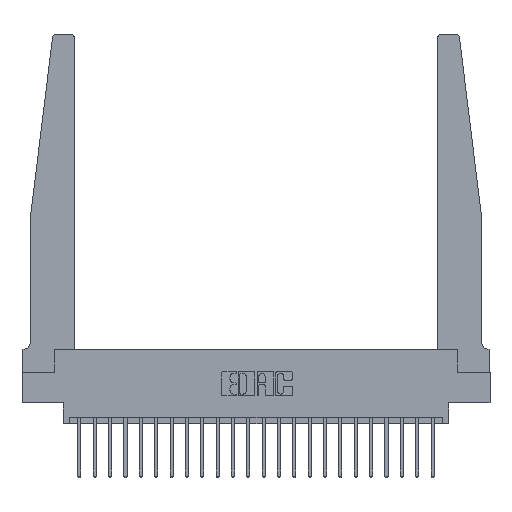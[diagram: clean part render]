
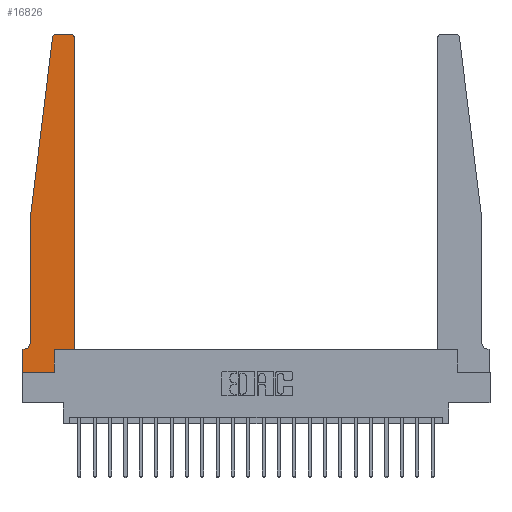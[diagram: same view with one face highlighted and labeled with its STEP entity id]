
A CAD part, top view. The second image highlights one B-rep face of the part: STEP entity #16826.
In plain terms, the highlighted planar face has unit normal (0, 0, 1).
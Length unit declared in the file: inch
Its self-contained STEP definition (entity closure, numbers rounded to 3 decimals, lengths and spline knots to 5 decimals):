
#52 = DIRECTION ( 'NONE',  ( -1., 0., 0. ) ) ;
#941 = EDGE_CURVE ( 'NONE', #4308, #5009, #6712, .T. ) ;
#975 = AXIS2_PLACEMENT_3D ( 'NONE', #16625, #5982, #18410 ) ;
#1387 = EDGE_CURVE ( 'NONE', #3531, #12288, #22010, .T. ) ;
#1699 = VECTOR ( 'NONE', #6866, 39.37008 ) ;
#2725 = VERTEX_POINT ( 'NONE', #20715 ) ;
#3095 = VECTOR ( 'NONE', #12484, 39.37008 ) ;
#3283 = LINE ( 'NONE', #10765, #21636 ) ;
#3531 = VERTEX_POINT ( 'NONE', #21065 ) ;
#3608 = EDGE_CURVE ( 'NONE', #15071, #17167, #10493, .T. ) ;
#3661 = CIRCLE ( 'NONE', #16187, 0.05 ) ;
#4035 = CARTESIAN_POINT ( 'NONE',  ( 0.2605, 0., 0.37 ) ) ;
#4235 = DIRECTION ( 'NONE',  ( 0., 0., 1. ) ) ;
#4308 = VERTEX_POINT ( 'NONE', #21750 ) ;
#4326 = CARTESIAN_POINT ( 'NONE',  ( 0.065, 0.1875, 0.37 ) ) ;
#4566 = DIRECTION ( 'NONE',  ( 0., 0., 1. ) ) ;
#4670 = CARTESIAN_POINT ( 'NONE',  ( 0.24675, 2.72367, 0.37 ) ) ;
#4792 = ORIENTED_EDGE ( 'NONE', *, *, #5842, .T. ) ;
#4995 = VECTOR ( 'NONE', #15937, 39.37008 ) ;
#5008 = CARTESIAN_POINT ( 'NONE',  ( 0.065, 0.2375, 0.37 ) ) ;
#5009 = VERTEX_POINT ( 'NONE', #4670 ) ;
#5294 = CARTESIAN_POINT ( 'NONE',  ( 0.2605, 0.18, 0.37 ) ) ;
#5448 = EDGE_CURVE ( 'NONE', #10392, #7543, #20905, .T. ) ;
#5519 = VECTOR ( 'NONE', #13654, 39.37008 ) ;
#5685 = EDGE_CURVE ( 'NONE', #8051, #8667, #15315, .T. ) ;
#5794 = ORIENTED_EDGE ( 'NONE', *, *, #17753, .T. ) ;
#5842 = EDGE_CURVE ( 'NONE', #12288, #10392, #3661, .T. ) ;
#5930 = CARTESIAN_POINT ( 'NONE',  ( 0., 0.1875, 0.37 ) ) ;
#5982 = DIRECTION ( 'NONE',  ( 0., 0., 1. ) ) ;
#6063 = ORIENTED_EDGE ( 'NONE', *, *, #5448, .T. ) ;
#6693 = CIRCLE ( 'NONE', #20726, 0.03 ) ;
#6712 = CIRCLE ( 'NONE', #975, 0.03 ) ;
#6866 = DIRECTION ( 'NONE',  ( -1., 0., 0. ) ) ;
#6918 = CARTESIAN_POINT ( 'NONE',  ( 0.2605, 0.18, 0.37 ) ) ;
#7245 = DIRECTION ( 'NONE',  ( 1., 0., 0. ) ) ;
#7543 = VERTEX_POINT ( 'NONE', #20799 ) ;
#7724 = AXIS2_PLACEMENT_3D ( 'NONE', #5930, #4235, #16647 ) ;
#8013 = EDGE_CURVE ( 'NONE', #17167, #8051, #3283, .T. ) ;
#8051 = VERTEX_POINT ( 'NONE', #16201 ) ;
#8667 = VERTEX_POINT ( 'NONE', #10658 ) ;
#8838 = DIRECTION ( 'NONE',  ( 0., 1., 0. ) ) ;
#10171 = ORIENTED_EDGE ( 'NONE', *, *, #17244, .T. ) ;
#10303 = CARTESIAN_POINT ( 'NONE',  ( 0.425, 0.18, 0.37 ) ) ;
#10392 = VERTEX_POINT ( 'NONE', #12357 ) ;
#10493 = LINE ( 'NONE', #5294, #19388 ) ;
#10658 = CARTESIAN_POINT ( 'NONE',  ( 0.425, 2.72, 0.37 ) ) ;
#10661 = CARTESIAN_POINT ( 'NONE',  ( 0., 0., 0.37 ) ) ;
#10682 = DIRECTION ( 'NONE',  ( 0., 0., -1. ) ) ;
#10765 = CARTESIAN_POINT ( 'NONE',  ( 0.425, 0.18, 0.37 ) ) ;
#12103 = ORIENTED_EDGE ( 'NONE', *, *, #18354, .T. ) ;
#12288 = VERTEX_POINT ( 'NONE', #5008 ) ;
#12357 = CARTESIAN_POINT ( 'NONE',  ( 0.015, 0.1875, 0.37 ) ) ;
#12484 = DIRECTION ( 'NONE',  ( 0., -1., 0. ) ) ;
#13575 = CARTESIAN_POINT ( 'NONE',  ( 0., 0., 0.37 ) ) ;
#13654 = DIRECTION ( 'NONE',  ( 1., 0., 0. ) ) ;
#14345 = ORIENTED_EDGE ( 'NONE', *, *, #22231, .T. ) ;
#14426 = LINE ( 'NONE', #10661, #4995 ) ;
#14865 = LINE ( 'NONE', #16550, #20190 ) ;
#14950 = LINE ( 'NONE', #13575, #5519 ) ;
#15071 = VERTEX_POINT ( 'NONE', #4035 ) ;
#15179 = CARTESIAN_POINT ( 'NONE',  ( 0.395, 2.72, 0.37 ) ) ;
#15315 = LINE ( 'NONE', #10303, #20073 ) ;
#15380 = VERTEX_POINT ( 'NONE', #19311 ) ;
#15612 = VECTOR ( 'NONE', #18534, 39.37008 ) ;
#15937 = DIRECTION ( 'NONE',  ( 0., -1., 0. ) ) ;
#16187 = AXIS2_PLACEMENT_3D ( 'NONE', #21339, #10682, #52 ) ;
#16201 = CARTESIAN_POINT ( 'NONE',  ( 0.425, 0.18, 0.37 ) ) ;
#16550 = CARTESIAN_POINT ( 'NONE',  ( 0.065, 1.25, 0.37 ) ) ;
#16625 = CARTESIAN_POINT ( 'NONE',  ( 0.27653, 2.72, 0.37 ) ) ;
#16647 = DIRECTION ( 'NONE',  ( 1., 0., 0. ) ) ;
#16826 = ADVANCED_FACE ( 'NONE', ( #18626 ), #21961, .T. ) ;
#16979 = LINE ( 'NONE', #19312, #1699 ) ;
#16988 = DIRECTION ( 'NONE',  ( 1., 0., 0. ) ) ;
#17167 = VERTEX_POINT ( 'NONE', #6918 ) ;
#17244 = EDGE_CURVE ( 'NONE', #7543, #15380, #14426, .T. ) ;
#17563 = ORIENTED_EDGE ( 'NONE', *, *, #1387, .T. ) ;
#17753 = EDGE_CURVE ( 'NONE', #15380, #15071, #14950, .T. ) ;
#17861 = CARTESIAN_POINT ( 'NONE',  ( 0.065, 1.25, 0.37 ) ) ;
#18340 = DIRECTION ( 'NONE',  ( -0.122, -0.992, 0. ) ) ;
#18354 = EDGE_CURVE ( 'NONE', #8667, #2725, #6693, .T. ) ;
#18410 = DIRECTION ( 'NONE',  ( 1., 0., 0. ) ) ;
#18534 = DIRECTION ( 'NONE',  ( -1., 0., 0. ) ) ;
#18574 = EDGE_CURVE ( 'NONE', #2725, #4308, #16979, .T. ) ;
#18626 = FACE_OUTER_BOUND ( 'NONE', #19400, .T. ) ;
#19311 = CARTESIAN_POINT ( 'NONE',  ( 0., 0., 0.37 ) ) ;
#19312 = CARTESIAN_POINT ( 'NONE',  ( 0.25, 2.75, 0.37 ) ) ;
#19388 = VECTOR ( 'NONE', #8838, 39.37008 ) ;
#19400 = EDGE_LOOP ( 'NONE', ( #21824, #20572, #14345, #17563, #4792, #6063, #10171, #5794, #21204, #19906, #20296, #12103 ) ) ;
#19906 = ORIENTED_EDGE ( 'NONE', *, *, #8013, .T. ) ;
#20073 = VECTOR ( 'NONE', #22756, 39.37008 ) ;
#20190 = VECTOR ( 'NONE', #18340, 39.37008 ) ;
#20296 = ORIENTED_EDGE ( 'NONE', *, *, #5685, .T. ) ;
#20572 = ORIENTED_EDGE ( 'NONE', *, *, #941, .T. ) ;
#20715 = CARTESIAN_POINT ( 'NONE',  ( 0.395, 2.75, 0.37 ) ) ;
#20726 = AXIS2_PLACEMENT_3D ( 'NONE', #15179, #4566, #16988 ) ;
#20799 = CARTESIAN_POINT ( 'NONE',  ( 0., 0.1875, 0.37 ) ) ;
#20905 = LINE ( 'NONE', #4326, #15612 ) ;
#21065 = CARTESIAN_POINT ( 'NONE',  ( 0.065, 1.25, 0.37 ) ) ;
#21204 = ORIENTED_EDGE ( 'NONE', *, *, #3608, .T. ) ;
#21339 = CARTESIAN_POINT ( 'NONE',  ( 0.015, 0.2375, 0.37 ) ) ;
#21636 = VECTOR ( 'NONE', #7245, 39.37008 ) ;
#21750 = CARTESIAN_POINT ( 'NONE',  ( 0.27653, 2.75, 0.37 ) ) ;
#21824 = ORIENTED_EDGE ( 'NONE', *, *, #18574, .T. ) ;
#21961 = PLANE ( 'NONE',  #7724 ) ;
#22010 = LINE ( 'NONE', #17861, #3095 ) ;
#22231 = EDGE_CURVE ( 'NONE', #5009, #3531, #14865, .T. ) ;
#22756 = DIRECTION ( 'NONE',  ( 0., 1., 0. ) ) ;
